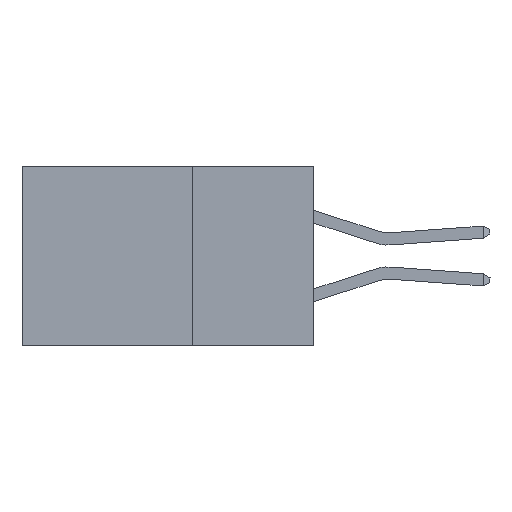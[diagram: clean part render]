
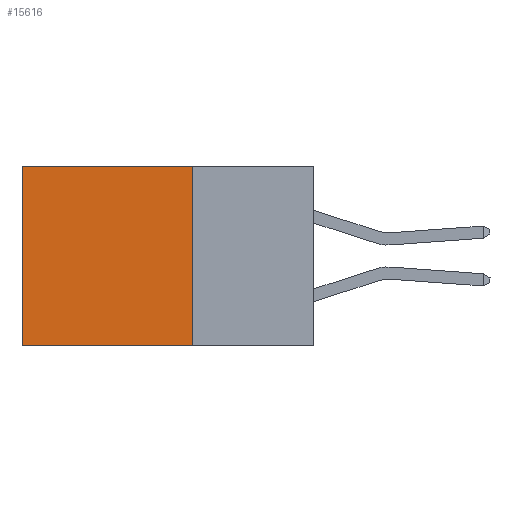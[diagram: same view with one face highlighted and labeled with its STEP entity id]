
A CAD part, left-side view. The second image highlights one B-rep face of the part: STEP entity #15616.
In plain terms, the highlighted planar face has unit normal (-1, 0, 0).
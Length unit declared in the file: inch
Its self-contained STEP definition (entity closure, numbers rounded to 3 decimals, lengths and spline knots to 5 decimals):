
#2018 = EDGE_CURVE ( 'NONE', #7561, #9255, #20227, .T. ) ;
#3033 = DIRECTION ( 'NONE',  ( 0., 0., -1. ) ) ;
#5283 = EDGE_LOOP ( 'NONE', ( #8590, #19828, #19961, #18147 ) ) ;
#5604 = DIRECTION ( 'NONE',  ( 0., 1., 0. ) ) ;
#5682 = CARTESIAN_POINT ( 'NONE',  ( 0.2875, 0.25, -0.37 ) ) ;
#5947 = VECTOR ( 'NONE', #17647, 39.37008 ) ;
#6333 = VECTOR ( 'NONE', #17587, 39.37008 ) ;
#6724 = EDGE_CURVE ( 'NONE', #14351, #12224, #10833, .T. ) ;
#7508 = CARTESIAN_POINT ( 'NONE',  ( 0.2875, 0.25, 0. ) ) ;
#7561 = VERTEX_POINT ( 'NONE', #19999 ) ;
#7750 = CARTESIAN_POINT ( 'NONE',  ( 0.2875, 0.6, -0.37 ) ) ;
#8590 = ORIENTED_EDGE ( 'NONE', *, *, #17304, .T. ) ;
#9213 = DIRECTION ( 'NONE',  ( 0., 0., -1. ) ) ;
#9255 = VERTEX_POINT ( 'NONE', #7750 ) ;
#10833 = LINE ( 'NONE', #15857, #6333 ) ;
#11476 = CARTESIAN_POINT ( 'NONE',  ( 0.2875, 0.25, 0. ) ) ;
#11490 = LINE ( 'NONE', #15923, #5947 ) ;
#12224 = VERTEX_POINT ( 'NONE', #20001 ) ;
#12909 = CARTESIAN_POINT ( 'NONE',  ( 0.2875, 0.25, 0. ) ) ;
#13143 = DIRECTION ( 'NONE',  ( 1., 0., 0. ) ) ;
#14222 = EDGE_CURVE ( 'NONE', #14351, #7561, #15770, .T. ) ;
#14351 = VERTEX_POINT ( 'NONE', #12909 ) ;
#15240 = VECTOR ( 'NONE', #9213, 39.37008 ) ;
#15616 = ADVANCED_FACE ( 'NONE', ( #21515 ), #19856, .F. ) ;
#15705 = VECTOR ( 'NONE', #5604, 39.37008 ) ;
#15770 = LINE ( 'NONE', #7508, #15240 ) ;
#15857 = CARTESIAN_POINT ( 'NONE',  ( 0.2875, 0.25, 0. ) ) ;
#15923 = CARTESIAN_POINT ( 'NONE',  ( 0.2875, 0.6, 0. ) ) ;
#17304 = EDGE_CURVE ( 'NONE', #12224, #9255, #11490, .T. ) ;
#17587 = DIRECTION ( 'NONE',  ( 0., 1., 0. ) ) ;
#17647 = DIRECTION ( 'NONE',  ( 0., 0., -1. ) ) ;
#18147 = ORIENTED_EDGE ( 'NONE', *, *, #6724, .T. ) ;
#19828 = ORIENTED_EDGE ( 'NONE', *, *, #2018, .F. ) ;
#19856 = PLANE ( 'NONE',  #21627 ) ;
#19961 = ORIENTED_EDGE ( 'NONE', *, *, #14222, .F. ) ;
#19999 = CARTESIAN_POINT ( 'NONE',  ( 0.2875, 0.25, -0.37 ) ) ;
#20001 = CARTESIAN_POINT ( 'NONE',  ( 0.2875, 0.6, 0. ) ) ;
#20227 = LINE ( 'NONE', #5682, #15705 ) ;
#21515 = FACE_OUTER_BOUND ( 'NONE', #5283, .T. ) ;
#21627 = AXIS2_PLACEMENT_3D ( 'NONE', #11476, #13143, #3033 ) ;
